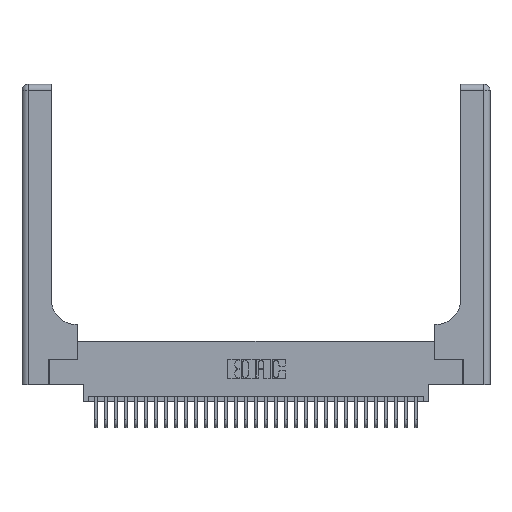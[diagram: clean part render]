
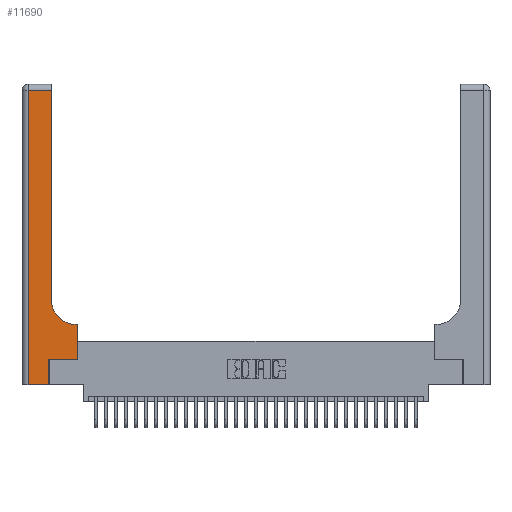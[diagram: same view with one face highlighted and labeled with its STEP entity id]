
A CAD part, top view. The second image highlights one B-rep face of the part: STEP entity #11690.
In plain terms, the highlighted planar face has unit normal (0, 0, 1).
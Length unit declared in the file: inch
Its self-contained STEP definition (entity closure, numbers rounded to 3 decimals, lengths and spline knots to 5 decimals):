
#457 = LINE ( 'NONE', #10438, #5456 ) ;
#600 = ORIENTED_EDGE ( 'NONE', *, *, #27235, .T. ) ;
#707 = DIRECTION ( 'NONE',  ( -1., 0., 0. ) ) ;
#1263 = ORIENTED_EDGE ( 'NONE', *, *, #23145, .T. ) ;
#1322 = ORIENTED_EDGE ( 'NONE', *, *, #10244, .T. ) ;
#1415 = CARTESIAN_POINT ( 'NONE',  ( 0.5415, 0.85, 0.37 ) ) ;
#1852 = EDGE_CURVE ( 'NONE', #14903, #10921, #3227, .T. ) ;
#2348 = CIRCLE ( 'NONE', #23961, 0.25 ) ;
#2646 = LINE ( 'NONE', #22532, #12741 ) ;
#2862 = ORIENTED_EDGE ( 'NONE', *, *, #29512, .T. ) ;
#3088 = EDGE_CURVE ( 'NONE', #3442, #8748, #7734, .T. ) ;
#3125 = DIRECTION ( 'NONE',  ( -1., 0., 0. ) ) ;
#3133 = EDGE_CURVE ( 'NONE', #10921, #28403, #457, .T. ) ;
#3227 = LINE ( 'NONE', #3929, #29796 ) ;
#3442 = VERTEX_POINT ( 'NONE', #23754 ) ;
#3736 = ORIENTED_EDGE ( 'NONE', *, *, #3088, .T. ) ;
#3899 = DIRECTION ( 'NONE',  ( 1., 0., 0. ) ) ;
#3929 = CARTESIAN_POINT ( 'NONE',  ( 0.5585, 0.25, 0.37 ) ) ;
#4006 = CARTESIAN_POINT ( 'NONE',  ( 0.2915, 3., 0.37 ) ) ;
#4157 = VERTEX_POINT ( 'NONE', #12391 ) ;
#4744 = PLANE ( 'NONE',  #23479 ) ;
#4870 = LINE ( 'NONE', #4886, #30644 ) ;
#4886 = CARTESIAN_POINT ( 'NONE',  ( 0.06, 3., 0.37 ) ) ;
#5456 = VECTOR ( 'NONE', #707, 39.37008 ) ;
#6795 = ORIENTED_EDGE ( 'NONE', *, *, #1852, .T. ) ;
#6985 = VECTOR ( 'NONE', #15116, 39.37008 ) ;
#7198 = DIRECTION ( 'NONE',  ( -1., 0., 0. ) ) ;
#7734 = LINE ( 'NONE', #22315, #6985 ) ;
#8156 = VECTOR ( 'NONE', #10275, 39.37008 ) ;
#8748 = VERTEX_POINT ( 'NONE', #12054 ) ;
#9390 = VECTOR ( 'NONE', #3125, 39.37008 ) ;
#10167 = LINE ( 'NONE', #17683, #9390 ) ;
#10234 = CARTESIAN_POINT ( 'NONE',  ( 0.5585, 0.25, 0.37 ) ) ;
#10244 = EDGE_CURVE ( 'NONE', #4157, #14431, #10167, .T. ) ;
#10275 = DIRECTION ( 'NONE',  ( 1., 0., 0. ) ) ;
#10438 = CARTESIAN_POINT ( 'NONE',  ( 0.2915, 0.6, 0.37 ) ) ;
#10921 = VERTEX_POINT ( 'NONE', #25665 ) ;
#11063 = VECTOR ( 'NONE', #11354, 39.37008 ) ;
#11354 = DIRECTION ( 'NONE',  ( 0., 1., 0. ) ) ;
#11690 = ADVANCED_FACE ( 'NONE', ( #24979 ), #4744, .F. ) ;
#11826 = LINE ( 'NONE', #4006, #11063 ) ;
#12054 = CARTESIAN_POINT ( 'NONE',  ( 0.269, 0., 0.37 ) ) ;
#12391 = CARTESIAN_POINT ( 'NONE',  ( 0.2915, 2.94, 0.37 ) ) ;
#12741 = VECTOR ( 'NONE', #29701, 39.37008 ) ;
#14302 = EDGE_CURVE ( 'NONE', #15574, #14903, #14616, .T. ) ;
#14431 = VERTEX_POINT ( 'NONE', #22876 ) ;
#14603 = CARTESIAN_POINT ( 'NONE',  ( 0.2915, 0.85, 0.37 ) ) ;
#14616 = LINE ( 'NONE', #19930, #8156 ) ;
#14903 = VERTEX_POINT ( 'NONE', #10234 ) ;
#15116 = DIRECTION ( 'NONE',  ( 1., 0., 0. ) ) ;
#15574 = VERTEX_POINT ( 'NONE', #18270 ) ;
#17683 = CARTESIAN_POINT ( 'NONE',  ( 0., 2.94, 0.37 ) ) ;
#17722 = VERTEX_POINT ( 'NONE', #14603 ) ;
#18270 = CARTESIAN_POINT ( 'NONE',  ( 0.269, 0.25, 0.37 ) ) ;
#18467 = DIRECTION ( 'NONE',  ( 0., 0., -1. ) ) ;
#18497 = DIRECTION ( 'NONE',  ( 0., 1., 0. ) ) ;
#19704 = ORIENTED_EDGE ( 'NONE', *, *, #3133, .T. ) ;
#19930 = CARTESIAN_POINT ( 'NONE',  ( 0.269, 0.25, 0.37 ) ) ;
#20943 = ORIENTED_EDGE ( 'NONE', *, *, #25670, .T. ) ;
#21061 = CARTESIAN_POINT ( 'NONE',  ( 0.5415, 0.6, 0.37 ) ) ;
#21725 = DIRECTION ( 'NONE',  ( 0., 0., -1. ) ) ;
#21766 = DIRECTION ( 'NONE',  ( 0., -1., 0. ) ) ;
#22315 = CARTESIAN_POINT ( 'NONE',  ( 0., 0., 0.37 ) ) ;
#22532 = CARTESIAN_POINT ( 'NONE',  ( 0.269, 0., 0.37 ) ) ;
#22876 = CARTESIAN_POINT ( 'NONE',  ( 0.06, 2.94, 0.37 ) ) ;
#23145 = EDGE_CURVE ( 'NONE', #8748, #15574, #2646, .T. ) ;
#23479 = AXIS2_PLACEMENT_3D ( 'NONE', #31324, #21725, #7198 ) ;
#23754 = CARTESIAN_POINT ( 'NONE',  ( 0.06, 0., 0.37 ) ) ;
#23915 = ORIENTED_EDGE ( 'NONE', *, *, #14302, .T. ) ;
#23961 = AXIS2_PLACEMENT_3D ( 'NONE', #1415, #18467, #3899 ) ;
#24979 = FACE_OUTER_BOUND ( 'NONE', #29509, .T. ) ;
#25665 = CARTESIAN_POINT ( 'NONE',  ( 0.5585, 0.6, 0.37 ) ) ;
#25670 = EDGE_CURVE ( 'NONE', #17722, #4157, #11826, .T. ) ;
#27235 = EDGE_CURVE ( 'NONE', #14431, #3442, #4870, .T. ) ;
#28403 = VERTEX_POINT ( 'NONE', #21061 ) ;
#29509 = EDGE_LOOP ( 'NONE', ( #20943, #1322, #600, #3736, #1263, #23915, #6795, #19704, #2862 ) ) ;
#29512 = EDGE_CURVE ( 'NONE', #28403, #17722, #2348, .T. ) ;
#29701 = DIRECTION ( 'NONE',  ( 0., 1., 0. ) ) ;
#29796 = VECTOR ( 'NONE', #18497, 39.37008 ) ;
#30644 = VECTOR ( 'NONE', #21766, 39.37008 ) ;
#31324 = CARTESIAN_POINT ( 'NONE',  ( 0., 3., 0.37 ) ) ;
